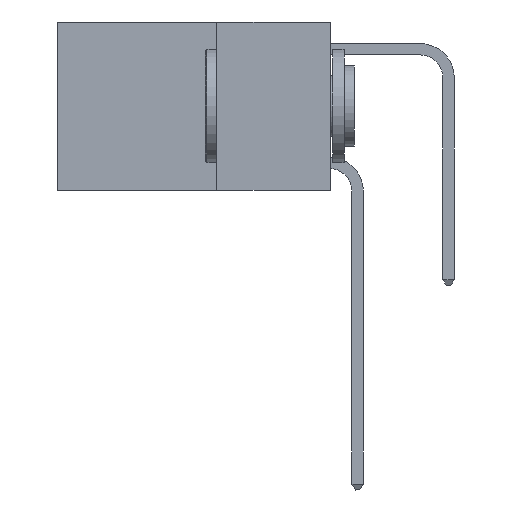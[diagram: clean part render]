
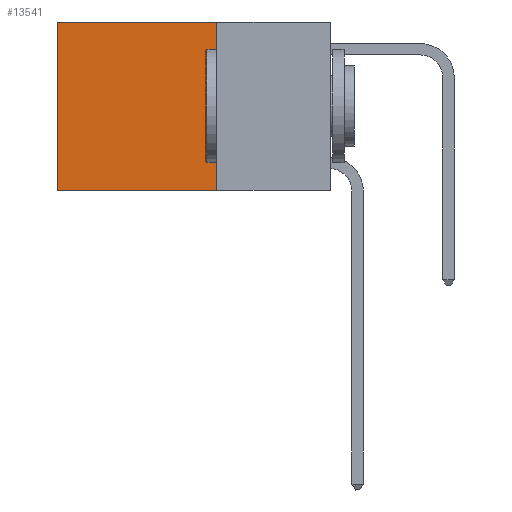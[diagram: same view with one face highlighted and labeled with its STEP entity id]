
A CAD part, left-side view. The second image highlights one B-rep face of the part: STEP entity #13541.
In plain terms, the highlighted planar face has unit normal (-1, 0, 0).
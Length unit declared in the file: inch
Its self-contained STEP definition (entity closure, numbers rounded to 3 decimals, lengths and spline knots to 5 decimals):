
#260 = FACE_OUTER_BOUND ( 'NONE', #11246, .T. ) ;
#1138 = CARTESIAN_POINT ( 'NONE',  ( 0.2625, 0.25, -0.37 ) ) ;
#2250 = CARTESIAN_POINT ( 'NONE',  ( 0.2625, 0.25, -0.37 ) ) ;
#3222 = EDGE_CURVE ( 'NONE', #8657, #10161, #10982, .T. ) ;
#3916 = LINE ( 'NONE', #1138, #7799 ) ;
#4064 = EDGE_CURVE ( 'NONE', #8657, #7108, #9180, .T. ) ;
#4944 = DIRECTION ( 'NONE',  ( 0., 0., -1. ) ) ;
#5067 = ORIENTED_EDGE ( 'NONE', *, *, #3222, .F. ) ;
#5628 = CARTESIAN_POINT ( 'NONE',  ( 0.2625, 0.25, 0. ) ) ;
#5760 = ORIENTED_EDGE ( 'NONE', *, *, #16839, .T. ) ;
#6378 = CARTESIAN_POINT ( 'NONE',  ( 0.2625, 0.25, 0. ) ) ;
#6707 = VERTEX_POINT ( 'NONE', #12641 ) ;
#7068 = LINE ( 'NONE', #11480, #9158 ) ;
#7108 = VERTEX_POINT ( 'NONE', #10993 ) ;
#7799 = VECTOR ( 'NONE', #14342, 39.37008 ) ;
#8657 = VERTEX_POINT ( 'NONE', #6378 ) ;
#9137 = PLANE ( 'NONE',  #12432 ) ;
#9158 = VECTOR ( 'NONE', #18764, 39.37008 ) ;
#9180 = LINE ( 'NONE', #9650, #17830 ) ;
#9650 = CARTESIAN_POINT ( 'NONE',  ( 0.2625, 0.25, 0. ) ) ;
#10161 = VERTEX_POINT ( 'NONE', #2250 ) ;
#10614 = EDGE_CURVE ( 'NONE', #10161, #6707, #3916, .T. ) ;
#10982 = LINE ( 'NONE', #16812, #13919 ) ;
#10993 = CARTESIAN_POINT ( 'NONE',  ( 0.2625, 0.6, 0. ) ) ;
#11246 = EDGE_LOOP ( 'NONE', ( #5760, #14580, #5067, #18625 ) ) ;
#11464 = DIRECTION ( 'NONE',  ( 1., 0., 0. ) ) ;
#11480 = CARTESIAN_POINT ( 'NONE',  ( 0.2625, 0.6, 0. ) ) ;
#12432 = AXIS2_PLACEMENT_3D ( 'NONE', #5628, #11464, #17693 ) ;
#12641 = CARTESIAN_POINT ( 'NONE',  ( 0.2625, 0.6, -0.37 ) ) ;
#13541 = ADVANCED_FACE ( 'NONE', ( #260 ), #9137, .F. ) ;
#13919 = VECTOR ( 'NONE', #4944, 39.37008 ) ;
#14342 = DIRECTION ( 'NONE',  ( 0., 1., 0. ) ) ;
#14580 = ORIENTED_EDGE ( 'NONE', *, *, #10614, .F. ) ;
#16812 = CARTESIAN_POINT ( 'NONE',  ( 0.2625, 0.25, 0. ) ) ;
#16839 = EDGE_CURVE ( 'NONE', #7108, #6707, #7068, .T. ) ;
#17693 = DIRECTION ( 'NONE',  ( 0., 0., -1. ) ) ;
#17830 = VECTOR ( 'NONE', #18193, 39.37008 ) ;
#18193 = DIRECTION ( 'NONE',  ( 0., 1., 0. ) ) ;
#18625 = ORIENTED_EDGE ( 'NONE', *, *, #4064, .T. ) ;
#18764 = DIRECTION ( 'NONE',  ( 0., 0., -1. ) ) ;
